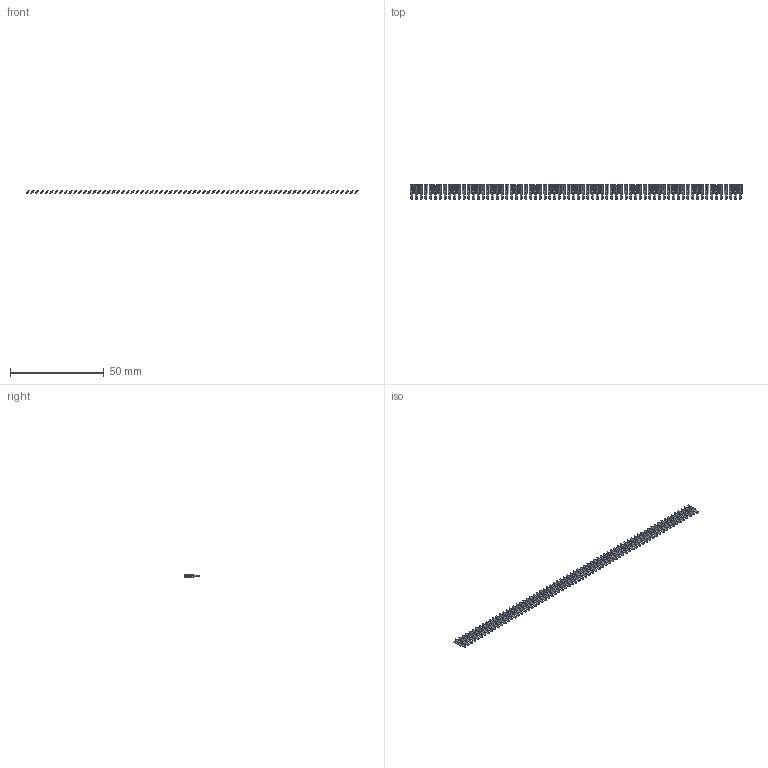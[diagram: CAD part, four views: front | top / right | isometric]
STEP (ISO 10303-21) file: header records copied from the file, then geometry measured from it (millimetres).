
FILE_DESCRIPTION (( 'STEP AP203' ), '1' );
FILE_NAME ('106-070-253-100.STEP', '2020-04-16T22:12:23', ( '' ), ( '' ), 'SwSTEP 2.0', 'SolidWorks 2016', '' );
FILE_SCHEMA (( 'CONFIG_CONTROL_DESIGN' ));
Length unit declared in the file: inch
Products named in the file (2): 100-290-001_100-290-253; 106-070-253-100
Assembly tree (70 placements, depth 2):
  106-070-253-100
    100-290-001_100-290-253  x70
Bounding box: 177.06 x 7.62 x 1.8 mm (x, y, z)
Volume: 386.2 mm3; surface area: 2408.5 mm2
Topology: 70 solids, 70 shells, 1400 faces, 3780 edges, 2520 vertices
Faces by surface type: plane 1330, cylinder 70
Entity records: 3028 total; most frequent: DIRECTION 242, CARTESIAN_POINT 183, CALENDAR_DATE 150, DATE_AND_TIME 150, LOCAL_TIME 150, COORDINATED_UNIVERSAL_TIME_OFFSET 150, ORIENTED_EDGE 108, AXIS2_PLACEMENT_3D 95
